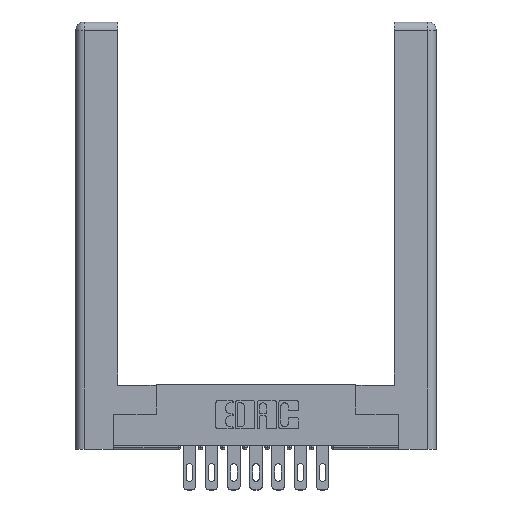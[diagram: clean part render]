
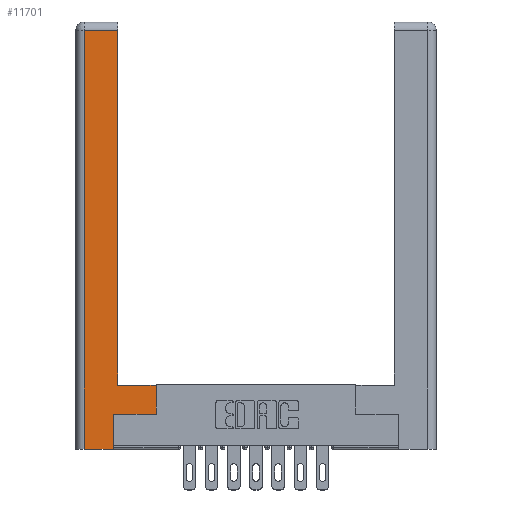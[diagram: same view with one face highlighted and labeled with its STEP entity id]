
A CAD part, top view. The second image highlights one B-rep face of the part: STEP entity #11701.
In plain terms, the highlighted planar face has unit normal (0, 0, 1).
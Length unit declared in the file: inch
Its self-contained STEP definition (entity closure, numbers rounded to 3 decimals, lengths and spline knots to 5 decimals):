
#124 = EDGE_CURVE ( 'NONE', #11535, #5166, #4507, .T. ) ;
#659 = CARTESIAN_POINT ( 'NONE',  ( 0.295, 3., 0. ) ) ;
#739 = VECTOR ( 'NONE', #1357, 39.37008 ) ;
#783 = VERTEX_POINT ( 'NONE', #3015 ) ;
#1038 = ORIENTED_EDGE ( 'NONE', *, *, #13883, .T. ) ;
#1335 = EDGE_CURVE ( 'NONE', #11485, #11535, #4098, .T. ) ;
#1349 = CARTESIAN_POINT ( 'NONE',  ( 0.565, 0.245, 0. ) ) ;
#1357 = DIRECTION ( 'NONE',  ( 0., 1., 0. ) ) ;
#1530 = CARTESIAN_POINT ( 'NONE',  ( 0., 0., 0. ) ) ;
#1573 = DIRECTION ( 'NONE',  ( -1., 0., 0. ) ) ;
#2183 = DIRECTION ( 'NONE',  ( -1., 0., 0. ) ) ;
#2207 = CARTESIAN_POINT ( 'NONE',  ( 0.0615, 0., 0. ) ) ;
#2645 = DIRECTION ( 'NONE',  ( 0., 0., -1. ) ) ;
#2803 = VECTOR ( 'NONE', #4720, 39.37008 ) ;
#2942 = ORIENTED_EDGE ( 'NONE', *, *, #13705, .T. ) ;
#2969 = DIRECTION ( 'NONE',  ( 0., -1., 0. ) ) ;
#3015 = CARTESIAN_POINT ( 'NONE',  ( 0.565, 0.245, 0. ) ) ;
#3078 = LINE ( 'NONE', #10958, #4675 ) ;
#3407 = EDGE_CURVE ( 'NONE', #783, #7733, #4929, .T. ) ;
#3598 = EDGE_CURVE ( 'NONE', #12349, #12537, #4579, .T. ) ;
#4098 = LINE ( 'NONE', #659, #739 ) ;
#4115 = CARTESIAN_POINT ( 'NONE',  ( 0.295, 0.45, 0. ) ) ;
#4131 = VECTOR ( 'NONE', #7729, 39.37008 ) ;
#4144 = LINE ( 'NONE', #1349, #4131 ) ;
#4507 = LINE ( 'NONE', #12366, #8171 ) ;
#4579 = LINE ( 'NONE', #5882, #2803 ) ;
#4675 = VECTOR ( 'NONE', #8690, 39.37008 ) ;
#4720 = DIRECTION ( 'NONE',  ( 1., 0., 0. ) ) ;
#4929 = LINE ( 'NONE', #7320, #14183 ) ;
#5166 = VERTEX_POINT ( 'NONE', #11446 ) ;
#5464 = ORIENTED_EDGE ( 'NONE', *, *, #13946, .T. ) ;
#5659 = CARTESIAN_POINT ( 'NONE',  ( 0.295, 2.94, 0. ) ) ;
#5705 = VERTEX_POINT ( 'NONE', #11845 ) ;
#5882 = CARTESIAN_POINT ( 'NONE',  ( 0.265, 0., 0. ) ) ;
#5936 = PLANE ( 'NONE',  #10971 ) ;
#6424 = VECTOR ( 'NONE', #2969, 39.37008 ) ;
#6777 = ORIENTED_EDGE ( 'NONE', *, *, #13359, .T. ) ;
#6853 = DIRECTION ( 'NONE',  ( -1., 0., 0. ) ) ;
#6937 = LINE ( 'NONE', #14055, #6424 ) ;
#7320 = CARTESIAN_POINT ( 'NONE',  ( 0.565, 0.45, 0. ) ) ;
#7368 = DIRECTION ( 'NONE',  ( 0., 1., 0. ) ) ;
#7729 = DIRECTION ( 'NONE',  ( 1., 0., 0. ) ) ;
#7733 = VERTEX_POINT ( 'NONE', #12736 ) ;
#8171 = VECTOR ( 'NONE', #2183, 39.37008 ) ;
#8345 = VECTOR ( 'NONE', #6853, 39.37008 ) ;
#8690 = DIRECTION ( 'NONE',  ( 0., 1., 0. ) ) ;
#8999 = ORIENTED_EDGE ( 'NONE', *, *, #124, .T. ) ;
#9043 = LINE ( 'NONE', #10173, #8345 ) ;
#9332 = CARTESIAN_POINT ( 'NONE',  ( 0.265, 0., 0. ) ) ;
#10173 = CARTESIAN_POINT ( 'NONE',  ( 0.295, 0.45, 0. ) ) ;
#10347 = ORIENTED_EDGE ( 'NONE', *, *, #3407, .T. ) ;
#10566 = EDGE_LOOP ( 'NONE', ( #12595, #8999, #2942, #13745, #1038, #5464, #10347, #6777 ) ) ;
#10958 = CARTESIAN_POINT ( 'NONE',  ( 0.265, 0.245, 0. ) ) ;
#10971 = AXIS2_PLACEMENT_3D ( 'NONE', #1530, #2645, #1573 ) ;
#11446 = CARTESIAN_POINT ( 'NONE',  ( 0.0615, 2.94, 0. ) ) ;
#11485 = VERTEX_POINT ( 'NONE', #4115 ) ;
#11535 = VERTEX_POINT ( 'NONE', #5659 ) ;
#11701 = ADVANCED_FACE ( 'NONE', ( #14198 ), #5936, .F. ) ;
#11845 = CARTESIAN_POINT ( 'NONE',  ( 0.265, 0.245, 0. ) ) ;
#12349 = VERTEX_POINT ( 'NONE', #2207 ) ;
#12366 = CARTESIAN_POINT ( 'NONE',  ( 0.0615, 2.94, 0. ) ) ;
#12537 = VERTEX_POINT ( 'NONE', #9332 ) ;
#12595 = ORIENTED_EDGE ( 'NONE', *, *, #1335, .T. ) ;
#12736 = CARTESIAN_POINT ( 'NONE',  ( 0.565, 0.45, 0. ) ) ;
#13359 = EDGE_CURVE ( 'NONE', #7733, #11485, #9043, .T. ) ;
#13705 = EDGE_CURVE ( 'NONE', #5166, #12349, #6937, .T. ) ;
#13745 = ORIENTED_EDGE ( 'NONE', *, *, #3598, .T. ) ;
#13883 = EDGE_CURVE ( 'NONE', #12537, #5705, #3078, .T. ) ;
#13946 = EDGE_CURVE ( 'NONE', #5705, #783, #4144, .T. ) ;
#14055 = CARTESIAN_POINT ( 'NONE',  ( 0.0615, 0., 0. ) ) ;
#14183 = VECTOR ( 'NONE', #7368, 39.37008 ) ;
#14198 = FACE_OUTER_BOUND ( 'NONE', #10566, .T. ) ;
